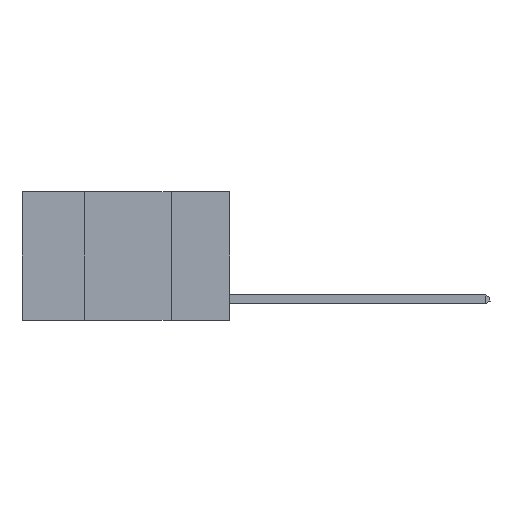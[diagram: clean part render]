
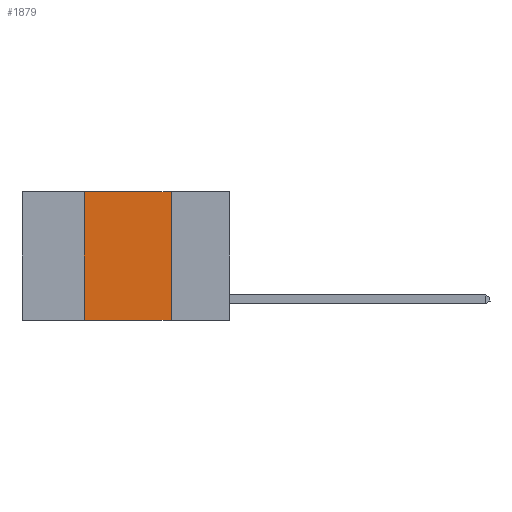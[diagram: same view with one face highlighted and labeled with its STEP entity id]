
A CAD part, left-side view. The second image highlights one B-rep face of the part: STEP entity #1879.
In plain terms, the highlighted planar face has unit normal (-1, 0, 0).
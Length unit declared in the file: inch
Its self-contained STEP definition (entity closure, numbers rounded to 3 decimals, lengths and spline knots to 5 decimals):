
#12 = LINE ( 'NONE', #5246, #8905 ) ;
#32 = EDGE_LOOP ( 'NONE', ( #8441, #5566, #7483, #6357 ) ) ;
#487 = CARTESIAN_POINT ( 'NONE',  ( 0., 0.17, -0.37 ) ) ;
#710 = EDGE_CURVE ( 'NONE', #3008, #2580, #7994, .T. ) ;
#1687 = CARTESIAN_POINT ( 'NONE',  ( 0., 0.17, 0. ) ) ;
#1879 = ADVANCED_FACE ( 'NONE', ( #2804 ), #7365, .F. ) ;
#1926 = DIRECTION ( 'NONE',  ( 1., 0., 0. ) ) ;
#2580 = VERTEX_POINT ( 'NONE', #487 ) ;
#2689 = CARTESIAN_POINT ( 'NONE',  ( 0., 0.6, -0.37 ) ) ;
#2804 = FACE_OUTER_BOUND ( 'NONE', #32, .T. ) ;
#2825 = VERTEX_POINT ( 'NONE', #7344 ) ;
#3008 = VERTEX_POINT ( 'NONE', #1687 ) ;
#3322 = CARTESIAN_POINT ( 'NONE',  ( 0., 0.6, 0. ) ) ;
#3503 = DIRECTION ( 'NONE',  ( 0., -1., 0. ) ) ;
#3541 = VECTOR ( 'NONE', #3503, 39.37008 ) ;
#3944 = CARTESIAN_POINT ( 'NONE',  ( 0., 0.6, 0. ) ) ;
#4107 = AXIS2_PLACEMENT_3D ( 'NONE', #3322, #1926, #8866 ) ;
#4563 = EDGE_CURVE ( 'NONE', #5913, #3008, #5712, .T. ) ;
#4695 = EDGE_CURVE ( 'NONE', #2825, #2580, #7826, .T. ) ;
#4942 = EDGE_CURVE ( 'NONE', #2825, #5913, #12, .T. ) ;
#5120 = DIRECTION ( 'NONE',  ( 0., 0., 1. ) ) ;
#5246 = CARTESIAN_POINT ( 'NONE',  ( 0., 0.42, 0. ) ) ;
#5566 = ORIENTED_EDGE ( 'NONE', *, *, #4563, .F. ) ;
#5583 = CARTESIAN_POINT ( 'NONE',  ( 0., 0.17, 0. ) ) ;
#5712 = LINE ( 'NONE', #3944, #7304 ) ;
#5913 = VERTEX_POINT ( 'NONE', #8249 ) ;
#6161 = VECTOR ( 'NONE', #8532, 39.37008 ) ;
#6357 = ORIENTED_EDGE ( 'NONE', *, *, #4695, .T. ) ;
#7304 = VECTOR ( 'NONE', #8929, 39.37008 ) ;
#7344 = CARTESIAN_POINT ( 'NONE',  ( 0., 0.42, -0.37 ) ) ;
#7365 = PLANE ( 'NONE',  #4107 ) ;
#7483 = ORIENTED_EDGE ( 'NONE', *, *, #4942, .F. ) ;
#7826 = LINE ( 'NONE', #2689, #3541 ) ;
#7994 = LINE ( 'NONE', #5583, #6161 ) ;
#8249 = CARTESIAN_POINT ( 'NONE',  ( 0., 0.42, 0. ) ) ;
#8441 = ORIENTED_EDGE ( 'NONE', *, *, #710, .F. ) ;
#8532 = DIRECTION ( 'NONE',  ( 0., 0., -1. ) ) ;
#8866 = DIRECTION ( 'NONE',  ( 0., 0., -1. ) ) ;
#8905 = VECTOR ( 'NONE', #5120, 39.37008 ) ;
#8929 = DIRECTION ( 'NONE',  ( 0., -1., 0. ) ) ;
